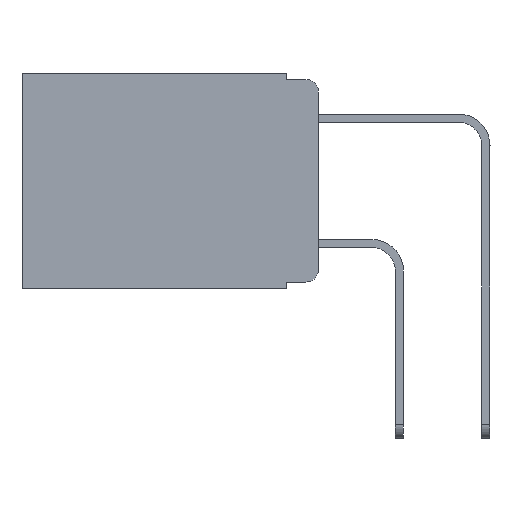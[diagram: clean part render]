
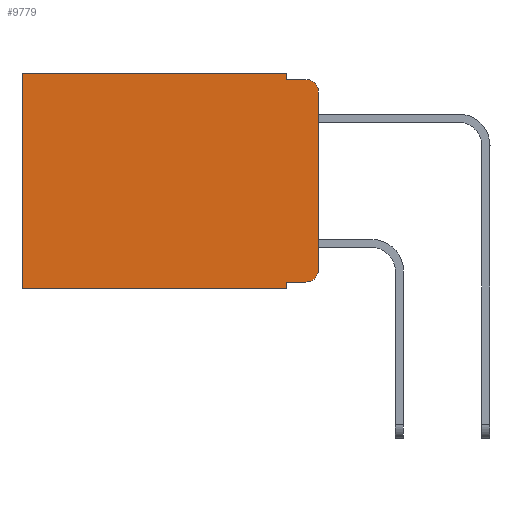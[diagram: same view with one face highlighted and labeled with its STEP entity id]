
A CAD part, left-side view. The second image highlights one B-rep face of the part: STEP entity #9779.
In plain terms, the highlighted planar face has unit normal (-1, 0, 0).
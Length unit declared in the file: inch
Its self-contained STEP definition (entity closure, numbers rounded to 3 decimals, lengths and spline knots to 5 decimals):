
#434 = EDGE_CURVE ( 'NONE', #9327, #6271, #9323, .T. ) ;
#652 = CARTESIAN_POINT ( 'NONE',  ( 0.298, 0.051, -0.343 ) ) ;
#798 = DIRECTION ( 'NONE',  ( 0., 0., -1. ) ) ;
#942 = DIRECTION ( 'NONE',  ( 0., 0., -1. ) ) ;
#950 = DIRECTION ( 'NONE',  ( 0., 1., 0. ) ) ;
#1141 = EDGE_CURVE ( 'NONE', #9327, #4769, #9908, .T. ) ;
#1305 = CARTESIAN_POINT ( 'NONE',  ( 0.298, 0.02, -0.03 ) ) ;
#1354 = LINE ( 'NONE', #10166, #9510 ) ;
#1573 = VECTOR ( 'NONE', #798, 39.37008 ) ;
#1701 = VERTEX_POINT ( 'NONE', #2451 ) ;
#1888 = DIRECTION ( 'NONE',  ( 0., 0., -1. ) ) ;
#2288 = ORIENTED_EDGE ( 'NONE', *, *, #9789, .F. ) ;
#2341 = EDGE_CURVE ( 'NONE', #5395, #6508, #1354, .T. ) ;
#2390 = CARTESIAN_POINT ( 'NONE',  ( 0.298, 0.02, -0.333 ) ) ;
#2430 = EDGE_LOOP ( 'NONE', ( #11289, #6199, #2288, #3321, #5817, #4076, #3290, #11617, #4914, #9340 ) ) ;
#2451 = CARTESIAN_POINT ( 'NONE',  ( 0.298, 0.473, 0. ) ) ;
#2522 = DIRECTION ( 'NONE',  ( 0., 0., -1. ) ) ;
#2526 = VECTOR ( 'NONE', #950, 39.37008 ) ;
#2575 = AXIS2_PLACEMENT_3D ( 'NONE', #6880, #2864, #1888 ) ;
#2585 = EDGE_CURVE ( 'NONE', #9373, #1701, #5122, .T. ) ;
#2864 = DIRECTION ( 'NONE',  ( 1., 0., 0. ) ) ;
#3199 = DIRECTION ( 'NONE',  ( 0., -1., 0. ) ) ;
#3290 = ORIENTED_EDGE ( 'NONE', *, *, #10196, .F. ) ;
#3321 = ORIENTED_EDGE ( 'NONE', *, *, #6913, .F. ) ;
#3727 = CARTESIAN_POINT ( 'NONE',  ( 0.298, 0.02, -0.313 ) ) ;
#3885 = PLANE ( 'NONE',  #2575 ) ;
#4047 = CARTESIAN_POINT ( 'NONE',  ( 0.298, 0.051, 0. ) ) ;
#4076 = ORIENTED_EDGE ( 'NONE', *, *, #8039, .T. ) ;
#4100 = LINE ( 'NONE', #8304, #9543 ) ;
#4123 = DIRECTION ( 'NONE',  ( 0., 0., -1. ) ) ;
#4162 = CARTESIAN_POINT ( 'NONE',  ( 0.298, 0.051, -0.333 ) ) ;
#4344 = EDGE_CURVE ( 'NONE', #6271, #6508, #6124, .T. ) ;
#4459 = CARTESIAN_POINT ( 'NONE',  ( 0.298, 0.051, -0.01 ) ) ;
#4465 = AXIS2_PLACEMENT_3D ( 'NONE', #1305, #8058, #9976 ) ;
#4769 = VERTEX_POINT ( 'NONE', #652 ) ;
#4914 = ORIENTED_EDGE ( 'NONE', *, *, #434, .T. ) ;
#5122 = LINE ( 'NONE', #11530, #2526 ) ;
#5395 = VERTEX_POINT ( 'NONE', #11301 ) ;
#5429 = VERTEX_POINT ( 'NONE', #10363 ) ;
#5492 = LINE ( 'NONE', #5601, #1573 ) ;
#5601 = CARTESIAN_POINT ( 'NONE',  ( 0.298, 0.473, 0. ) ) ;
#5817 = ORIENTED_EDGE ( 'NONE', *, *, #2585, .T. ) ;
#5820 = CARTESIAN_POINT ( 'NONE',  ( 0.298, 0.051, -0.01 ) ) ;
#5909 = DIRECTION ( 'NONE',  ( 0., -1., 0. ) ) ;
#6124 = CIRCLE ( 'NONE', #9745, 0.02 ) ;
#6199 = ORIENTED_EDGE ( 'NONE', *, *, #12393, .T. ) ;
#6271 = VERTEX_POINT ( 'NONE', #2390 ) ;
#6508 = VERTEX_POINT ( 'NONE', #12428 ) ;
#6527 = CARTESIAN_POINT ( 'NONE',  ( 0.298, 0.051, -0.333 ) ) ;
#6880 = CARTESIAN_POINT ( 'NONE',  ( 0.298, 0., 0. ) ) ;
#6913 = EDGE_CURVE ( 'NONE', #9373, #11935, #8970, .T. ) ;
#6995 = FACE_OUTER_BOUND ( 'NONE', #2430, .T. ) ;
#7623 = DIRECTION ( 'NONE',  ( -1., 0., 0. ) ) ;
#7971 = VECTOR ( 'NONE', #11581, 39.37008 ) ;
#8039 = EDGE_CURVE ( 'NONE', #1701, #8583, #5492, .T. ) ;
#8058 = DIRECTION ( 'NONE',  ( -1., 0., 0. ) ) ;
#8304 = CARTESIAN_POINT ( 'NONE',  ( 0.298, 0., -0.343 ) ) ;
#8517 = CARTESIAN_POINT ( 'NONE',  ( 0.298, 0.051, 0. ) ) ;
#8583 = VERTEX_POINT ( 'NONE', #10850 ) ;
#8659 = LINE ( 'NONE', #5820, #11812 ) ;
#8970 = LINE ( 'NONE', #4047, #11210 ) ;
#9323 = LINE ( 'NONE', #4162, #11134 ) ;
#9327 = VERTEX_POINT ( 'NONE', #6527 ) ;
#9340 = ORIENTED_EDGE ( 'NONE', *, *, #4344, .T. ) ;
#9373 = VERTEX_POINT ( 'NONE', #10319 ) ;
#9510 = VECTOR ( 'NONE', #2522, 39.37008 ) ;
#9543 = VECTOR ( 'NONE', #11342, 39.37008 ) ;
#9745 = AXIS2_PLACEMENT_3D ( 'NONE', #3727, #7623, #942 ) ;
#9779 = ADVANCED_FACE ( 'NONE', ( #6995 ), #3885, .F. ) ;
#9789 = EDGE_CURVE ( 'NONE', #11935, #5429, #8659, .T. ) ;
#9908 = LINE ( 'NONE', #8517, #7971 ) ;
#9976 = DIRECTION ( 'NONE',  ( 0., 0., -1. ) ) ;
#10166 = CARTESIAN_POINT ( 'NONE',  ( 0.298, 0., 0. ) ) ;
#10196 = EDGE_CURVE ( 'NONE', #4769, #8583, #4100, .T. ) ;
#10319 = CARTESIAN_POINT ( 'NONE',  ( 0.298, 0.051, 0. ) ) ;
#10363 = CARTESIAN_POINT ( 'NONE',  ( 0.298, 0.02, -0.01 ) ) ;
#10850 = CARTESIAN_POINT ( 'NONE',  ( 0.298, 0.473, -0.343 ) ) ;
#11134 = VECTOR ( 'NONE', #3199, 39.37008 ) ;
#11210 = VECTOR ( 'NONE', #4123, 39.37008 ) ;
#11289 = ORIENTED_EDGE ( 'NONE', *, *, #2341, .F. ) ;
#11301 = CARTESIAN_POINT ( 'NONE',  ( 0.298, 0., -0.03 ) ) ;
#11342 = DIRECTION ( 'NONE',  ( 0., 1., 0. ) ) ;
#11530 = CARTESIAN_POINT ( 'NONE',  ( 0.298, 0., 0. ) ) ;
#11581 = DIRECTION ( 'NONE',  ( 0., 0., -1. ) ) ;
#11612 = CIRCLE ( 'NONE', #4465, 0.02 ) ;
#11617 = ORIENTED_EDGE ( 'NONE', *, *, #1141, .F. ) ;
#11812 = VECTOR ( 'NONE', #5909, 39.37008 ) ;
#11935 = VERTEX_POINT ( 'NONE', #4459 ) ;
#12393 = EDGE_CURVE ( 'NONE', #5395, #5429, #11612, .T. ) ;
#12428 = CARTESIAN_POINT ( 'NONE',  ( 0.298, 0., -0.313 ) ) ;
